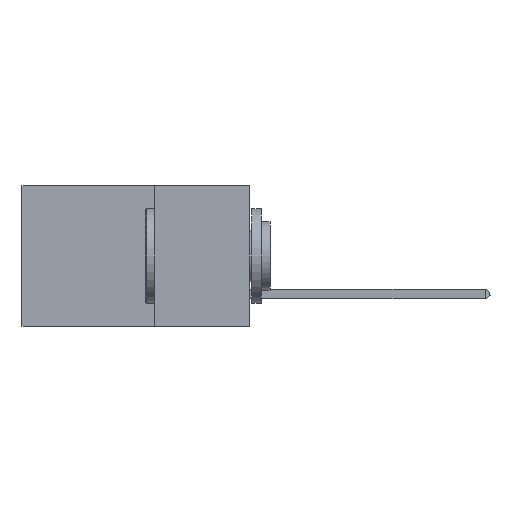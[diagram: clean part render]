
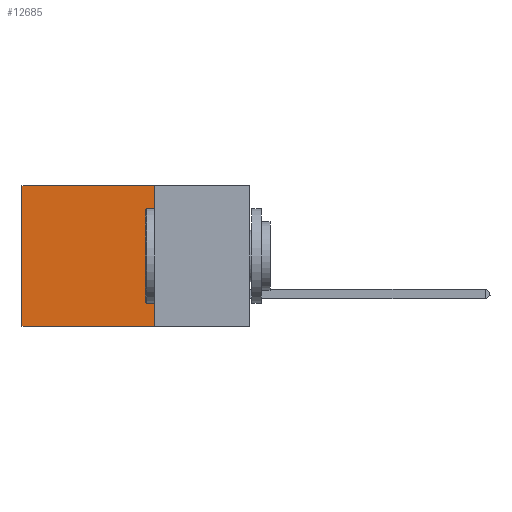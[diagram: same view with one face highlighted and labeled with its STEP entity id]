
A CAD part, left-side view. The second image highlights one B-rep face of the part: STEP entity #12685.
In plain terms, the highlighted planar face has unit normal (-1, 0, 0).
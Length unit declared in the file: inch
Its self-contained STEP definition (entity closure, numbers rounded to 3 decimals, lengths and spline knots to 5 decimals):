
#49 = VERTEX_POINT ( 'NONE', #2637 ) ;
#115 = CARTESIAN_POINT ( 'NONE',  ( 0.2875, 0.6, 0. ) ) ;
#485 = VERTEX_POINT ( 'NONE', #634 ) ;
#634 = CARTESIAN_POINT ( 'NONE',  ( 0.2875, 0.25, -0.37 ) ) ;
#1666 = ORIENTED_EDGE ( 'NONE', *, *, #12984, .F. ) ;
#2308 = CARTESIAN_POINT ( 'NONE',  ( 0.2875, 0.25, 0. ) ) ;
#2634 = CARTESIAN_POINT ( 'NONE',  ( 0.2875, 0.6, -0.37 ) ) ;
#2637 = CARTESIAN_POINT ( 'NONE',  ( 0.2875, 0.6, 0. ) ) ;
#2698 = VECTOR ( 'NONE', #12764, 39.37008 ) ;
#3224 = LINE ( 'NONE', #12711, #2698 ) ;
#3383 = DIRECTION ( 'NONE',  ( 0., 0., -1. ) ) ;
#4961 = CARTESIAN_POINT ( 'NONE',  ( 0.2875, 0.25, 0. ) ) ;
#6265 = EDGE_CURVE ( 'NONE', #12825, #49, #7675, .T. ) ;
#6273 = ORIENTED_EDGE ( 'NONE', *, *, #6743, .F. ) ;
#6743 = EDGE_CURVE ( 'NONE', #485, #7442, #3224, .T. ) ;
#7079 = VECTOR ( 'NONE', #3383, 39.37008 ) ;
#7283 = DIRECTION ( 'NONE',  ( 1., 0., 0. ) ) ;
#7442 = VERTEX_POINT ( 'NONE', #2634 ) ;
#7563 = LINE ( 'NONE', #2308, #7079 ) ;
#7675 = LINE ( 'NONE', #10333, #8693 ) ;
#7812 = EDGE_LOOP ( 'NONE', ( #13528, #6273, #1666, #10814 ) ) ;
#8259 = DIRECTION ( 'NONE',  ( 0., 1., 0. ) ) ;
#8693 = VECTOR ( 'NONE', #8259, 39.37008 ) ;
#8973 = LINE ( 'NONE', #115, #12813 ) ;
#9984 = EDGE_CURVE ( 'NONE', #49, #7442, #8973, .T. ) ;
#10333 = CARTESIAN_POINT ( 'NONE',  ( 0.2875, 0.25, 0. ) ) ;
#10452 = PLANE ( 'NONE',  #13045 ) ;
#10727 = FACE_OUTER_BOUND ( 'NONE', #7812, .T. ) ;
#10814 = ORIENTED_EDGE ( 'NONE', *, *, #6265, .T. ) ;
#11448 = DIRECTION ( 'NONE',  ( 0., 0., -1. ) ) ;
#12275 = DIRECTION ( 'NONE',  ( 0., 0., -1. ) ) ;
#12685 = ADVANCED_FACE ( 'NONE', ( #10727 ), #10452, .F. ) ;
#12711 = CARTESIAN_POINT ( 'NONE',  ( 0.2875, 0.25, -0.37 ) ) ;
#12764 = DIRECTION ( 'NONE',  ( 0., 1., 0. ) ) ;
#12813 = VECTOR ( 'NONE', #12275, 39.37008 ) ;
#12825 = VERTEX_POINT ( 'NONE', #4961 ) ;
#12984 = EDGE_CURVE ( 'NONE', #12825, #485, #7563, .T. ) ;
#13045 = AXIS2_PLACEMENT_3D ( 'NONE', #13465, #7283, #11448 ) ;
#13465 = CARTESIAN_POINT ( 'NONE',  ( 0.2875, 0.25, 0. ) ) ;
#13528 = ORIENTED_EDGE ( 'NONE', *, *, #9984, .T. ) ;
